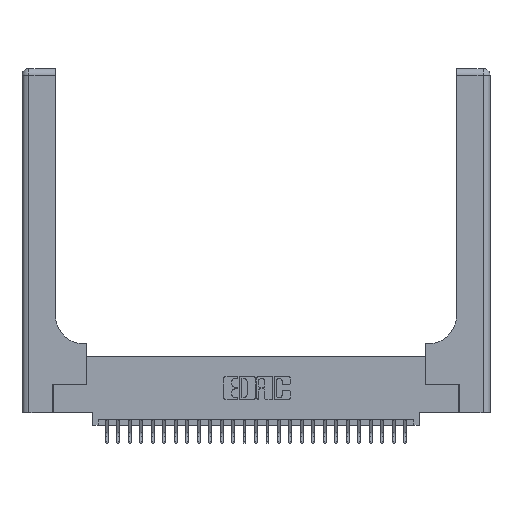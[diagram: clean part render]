
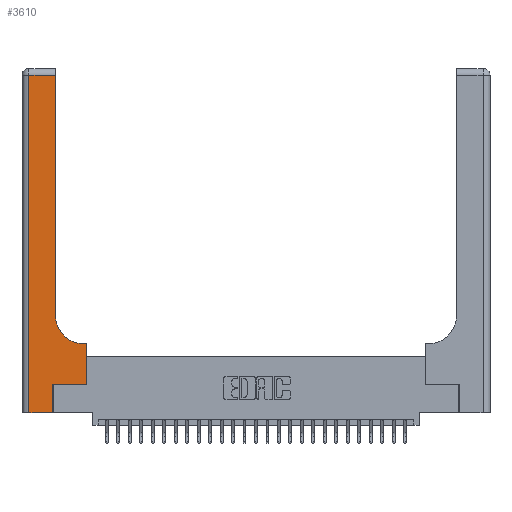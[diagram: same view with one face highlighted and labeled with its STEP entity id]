
A CAD part, top view. The second image highlights one B-rep face of the part: STEP entity #3610.
In plain terms, the highlighted planar face has unit normal (0, 0, 1).
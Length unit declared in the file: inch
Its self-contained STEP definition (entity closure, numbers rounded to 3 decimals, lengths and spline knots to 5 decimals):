
#12 = CARTESIAN_POINT ( 'NONE',  ( 0.269, 0., 0.37 ) ) ;
#63 = VERTEX_POINT ( 'NONE', #27664 ) ;
#722 = CARTESIAN_POINT ( 'NONE',  ( 0.06, 0., 0.37 ) ) ;
#1474 = ORIENTED_EDGE ( 'NONE', *, *, #17182, .T. ) ;
#1711 = ORIENTED_EDGE ( 'NONE', *, *, #4239, .T. ) ;
#1819 = EDGE_CURVE ( 'NONE', #24758, #25349, #18800, .T. ) ;
#2140 = LINE ( 'NONE', #2583, #18466 ) ;
#2561 = EDGE_CURVE ( 'NONE', #25349, #8121, #13527, .T. ) ;
#2583 = CARTESIAN_POINT ( 'NONE',  ( 0.2915, 3., 0.37 ) ) ;
#2835 = EDGE_CURVE ( 'NONE', #17044, #26593, #20847, .T. ) ;
#3610 = ADVANCED_FACE ( 'NONE', ( #13140 ), #4729, .F. ) ;
#4239 = EDGE_CURVE ( 'NONE', #19981, #63, #12760, .T. ) ;
#4729 = PLANE ( 'NONE',  #21656 ) ;
#4771 = DIRECTION ( 'NONE',  ( 0., 1., 0. ) ) ;
#6598 = VECTOR ( 'NONE', #20329, 39.37008 ) ;
#7470 = EDGE_LOOP ( 'NONE', ( #24456, #14363, #10922, #22221, #17361, #1474, #24728, #1711, #11424 ) ) ;
#7698 = AXIS2_PLACEMENT_3D ( 'NONE', #13017, #15183, #15278 ) ;
#7889 = CARTESIAN_POINT ( 'NONE',  ( 0.269, 0., 0.37 ) ) ;
#8121 = VERTEX_POINT ( 'NONE', #722 ) ;
#8866 = CIRCLE ( 'NONE', #7698, 0.25 ) ;
#9420 = VECTOR ( 'NONE', #13168, 39.37008 ) ;
#10359 = CARTESIAN_POINT ( 'NONE',  ( 0., 0., 0.37 ) ) ;
#10922 = ORIENTED_EDGE ( 'NONE', *, *, #2561, .T. ) ;
#11377 = CARTESIAN_POINT ( 'NONE',  ( 0.269, 0.25, 0.37 ) ) ;
#11424 = ORIENTED_EDGE ( 'NONE', *, *, #14489, .T. ) ;
#11791 = LINE ( 'NONE', #14010, #20500 ) ;
#11879 = VECTOR ( 'NONE', #17638, 39.37008 ) ;
#12760 = LINE ( 'NONE', #14328, #24551 ) ;
#13017 = CARTESIAN_POINT ( 'NONE',  ( 0.5415, 0.85, 0.37 ) ) ;
#13140 = FACE_OUTER_BOUND ( 'NONE', #7470, .T. ) ;
#13168 = DIRECTION ( 'NONE',  ( -1., 0., 0. ) ) ;
#13527 = LINE ( 'NONE', #15854, #6598 ) ;
#13678 = VERTEX_POINT ( 'NONE', #25971 ) ;
#13939 = LINE ( 'NONE', #22252, #11879 ) ;
#14010 = CARTESIAN_POINT ( 'NONE',  ( 0.5585, 0.25, 0.37 ) ) ;
#14129 = DIRECTION ( 'NONE',  ( -1., 0., 0. ) ) ;
#14328 = CARTESIAN_POINT ( 'NONE',  ( 0.2915, 0.6, 0.37 ) ) ;
#14363 = ORIENTED_EDGE ( 'NONE', *, *, #1819, .T. ) ;
#14439 = VECTOR ( 'NONE', #23460, 39.37008 ) ;
#14489 = EDGE_CURVE ( 'NONE', #63, #13678, #8866, .T. ) ;
#15170 = LINE ( 'NONE', #10359, #14439 ) ;
#15183 = DIRECTION ( 'NONE',  ( 0., 0., -1. ) ) ;
#15278 = DIRECTION ( 'NONE',  ( 1., 0., 0. ) ) ;
#15854 = CARTESIAN_POINT ( 'NONE',  ( 0.06, 3., 0.37 ) ) ;
#16059 = CARTESIAN_POINT ( 'NONE',  ( 0., 3., 0.37 ) ) ;
#16255 = DIRECTION ( 'NONE',  ( 0., 0., -1. ) ) ;
#16333 = VECTOR ( 'NONE', #27986, 39.37008 ) ;
#16465 = DIRECTION ( 'NONE',  ( 0., 1., 0. ) ) ;
#17044 = VERTEX_POINT ( 'NONE', #12 ) ;
#17182 = EDGE_CURVE ( 'NONE', #26593, #28539, #13939, .T. ) ;
#17361 = ORIENTED_EDGE ( 'NONE', *, *, #2835, .T. ) ;
#17508 = CARTESIAN_POINT ( 'NONE',  ( 0.5585, 0.25, 0.37 ) ) ;
#17638 = DIRECTION ( 'NONE',  ( 1., 0., 0. ) ) ;
#17864 = EDGE_CURVE ( 'NONE', #13678, #24758, #2140, .T. ) ;
#18338 = EDGE_CURVE ( 'NONE', #28539, #19981, #11791, .T. ) ;
#18466 = VECTOR ( 'NONE', #4771, 39.37008 ) ;
#18595 = DIRECTION ( 'NONE',  ( -1., 0., 0. ) ) ;
#18800 = LINE ( 'NONE', #24436, #9420 ) ;
#19981 = VERTEX_POINT ( 'NONE', #24537 ) ;
#20329 = DIRECTION ( 'NONE',  ( 0., -1., 0. ) ) ;
#20497 = CARTESIAN_POINT ( 'NONE',  ( 0.06, 2.94, 0.37 ) ) ;
#20500 = VECTOR ( 'NONE', #16465, 39.37008 ) ;
#20847 = LINE ( 'NONE', #7889, #16333 ) ;
#21656 = AXIS2_PLACEMENT_3D ( 'NONE', #16059, #16255, #18595 ) ;
#22221 = ORIENTED_EDGE ( 'NONE', *, *, #23178, .T. ) ;
#22252 = CARTESIAN_POINT ( 'NONE',  ( 0.269, 0.25, 0.37 ) ) ;
#23178 = EDGE_CURVE ( 'NONE', #8121, #17044, #15170, .T. ) ;
#23460 = DIRECTION ( 'NONE',  ( 1., 0., 0. ) ) ;
#24436 = CARTESIAN_POINT ( 'NONE',  ( 0., 2.94, 0.37 ) ) ;
#24456 = ORIENTED_EDGE ( 'NONE', *, *, #17864, .T. ) ;
#24537 = CARTESIAN_POINT ( 'NONE',  ( 0.5585, 0.6, 0.37 ) ) ;
#24551 = VECTOR ( 'NONE', #14129, 39.37008 ) ;
#24630 = CARTESIAN_POINT ( 'NONE',  ( 0.2915, 2.94, 0.37 ) ) ;
#24728 = ORIENTED_EDGE ( 'NONE', *, *, #18338, .T. ) ;
#24758 = VERTEX_POINT ( 'NONE', #24630 ) ;
#25349 = VERTEX_POINT ( 'NONE', #20497 ) ;
#25971 = CARTESIAN_POINT ( 'NONE',  ( 0.2915, 0.85, 0.37 ) ) ;
#26593 = VERTEX_POINT ( 'NONE', #11377 ) ;
#27664 = CARTESIAN_POINT ( 'NONE',  ( 0.5415, 0.6, 0.37 ) ) ;
#27986 = DIRECTION ( 'NONE',  ( 0., 1., 0. ) ) ;
#28539 = VERTEX_POINT ( 'NONE', #17508 ) ;
